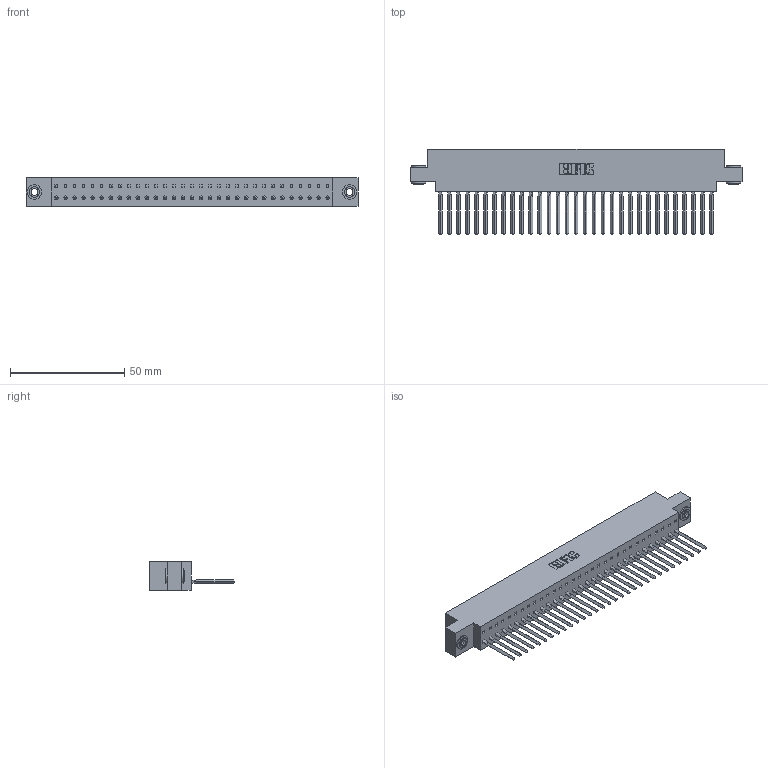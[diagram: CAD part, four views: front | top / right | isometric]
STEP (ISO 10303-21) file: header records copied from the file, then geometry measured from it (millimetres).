
FILE_DESCRIPTION (( 'STEP AP203' ), '1' );
FILE_NAME ('317-031-541-603.STEP', '2020-02-27T20:46:08', ( '' ), ( '' ), 'SwSTEP 2.0', 'SolidWorks 2016', '' );
FILE_SCHEMA (( 'CONFIG_CONTROL_DESIGN' ));
Length unit declared in the file: inch
Products named in the file (4): 317 Part_.156 Dia - TH; 317-290-002_541; 317-031-541-603; 345-250-002_345-250-002-102
Assembly tree (34 placements, depth 2):
  317-031-541-603
    317 Part_.156 Dia - TH
    317-290-002_541  x31
    345-250-002_345-250-002-102  x2
Bounding box: 145.54 x 37.34 x 12.7 mm (x, y, z)
Volume: 23283.2 mm3; surface area: 32748.6 mm2
Topology: 34 solids, 34 shells, 4852 faces, 13805 edges, 8972 vertices
Faces by surface type: plane 3912, cylinder 808, bspline 124, cone 8
Entity records: 47551 total; most frequent: CARTESIAN_POINT 9057, ORIENTED_EDGE 8334, DIRECTION 6879, EDGE_CURVE 4167, VECTOR 3779, LINE 3779, VERTEX_POINT 2768, AXIS2_PLACEMENT_3D 1550
